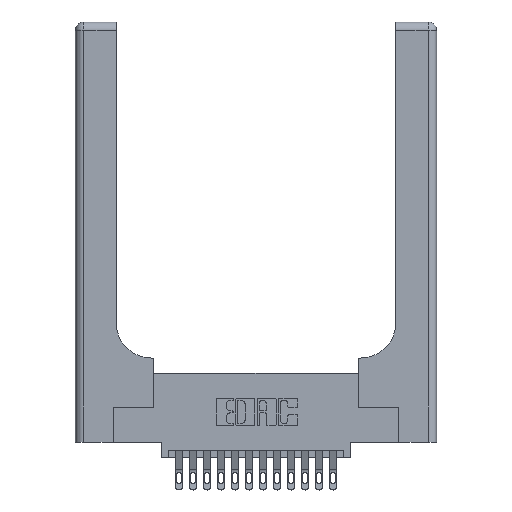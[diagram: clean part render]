
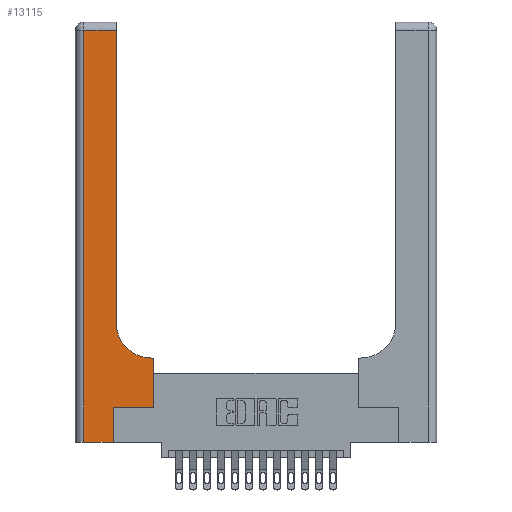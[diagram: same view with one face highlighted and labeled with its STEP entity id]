
A CAD part, top view. The second image highlights one B-rep face of the part: STEP entity #13115.
In plain terms, the highlighted planar face has unit normal (0, 0, 1).
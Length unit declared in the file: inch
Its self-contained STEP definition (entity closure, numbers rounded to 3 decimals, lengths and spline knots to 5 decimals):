
#173 = EDGE_CURVE ( 'NONE', #11766, #14935, #10008, .T. ) ;
#543 = ORIENTED_EDGE ( 'NONE', *, *, #10505, .T. ) ;
#1247 = CARTESIAN_POINT ( 'NONE',  ( 0.5415, 0.85, 0.37 ) ) ;
#1340 = VECTOR ( 'NONE', #4042, 39.37008 ) ;
#1445 = VECTOR ( 'NONE', #12052, 39.37008 ) ;
#2029 = FACE_OUTER_BOUND ( 'NONE', #12552, .T. ) ;
#2255 = EDGE_CURVE ( 'NONE', #11863, #18431, #16213, .T. ) ;
#2437 = CARTESIAN_POINT ( 'NONE',  ( 0.5415, 0.6, 0.37 ) ) ;
#2959 = AXIS2_PLACEMENT_3D ( 'NONE', #1247, #5546, #6904 ) ;
#3194 = CARTESIAN_POINT ( 'NONE',  ( 0., 0., 0.37 ) ) ;
#3254 = EDGE_CURVE ( 'NONE', #19071, #11415, #4834, .T. ) ;
#3651 = EDGE_CURVE ( 'NONE', #17172, #5859, #17070, .T. ) ;
#3893 = DIRECTION ( 'NONE',  ( 0., -1., 0. ) ) ;
#4042 = DIRECTION ( 'NONE',  ( 0., 1., 0. ) ) ;
#4176 = CARTESIAN_POINT ( 'NONE',  ( 0.06, 2.94, 0.37 ) ) ;
#4649 = DIRECTION ( 'NONE',  ( 1., 0., 0. ) ) ;
#4834 = LINE ( 'NONE', #18216, #10853 ) ;
#5546 = DIRECTION ( 'NONE',  ( 0., 0., -1. ) ) ;
#5724 = LINE ( 'NONE', #3194, #14033 ) ;
#5859 = VERTEX_POINT ( 'NONE', #2437 ) ;
#6064 = PLANE ( 'NONE',  #14473 ) ;
#6672 = CARTESIAN_POINT ( 'NONE',  ( 0.269, 0., 0.37 ) ) ;
#6705 = CARTESIAN_POINT ( 'NONE',  ( 0.269, 0.25, 0.37 ) ) ;
#6874 = CARTESIAN_POINT ( 'NONE',  ( 0.06, 3., 0.37 ) ) ;
#6904 = DIRECTION ( 'NONE',  ( 1., 0., 0. ) ) ;
#7171 = DIRECTION ( 'NONE',  ( -1., 0., 0. ) ) ;
#7426 = LINE ( 'NONE', #9111, #1445 ) ;
#9111 = CARTESIAN_POINT ( 'NONE',  ( 0., 2.94, 0.37 ) ) ;
#9123 = LINE ( 'NONE', #15254, #11876 ) ;
#9161 = VERTEX_POINT ( 'NONE', #6672 ) ;
#9186 = CARTESIAN_POINT ( 'NONE',  ( 0.2915, 2.94, 0.37 ) ) ;
#9344 = ORIENTED_EDGE ( 'NONE', *, *, #15703, .T. ) ;
#10008 = LINE ( 'NONE', #6705, #10236 ) ;
#10175 = VECTOR ( 'NONE', #7171, 39.37008 ) ;
#10236 = VECTOR ( 'NONE', #12768, 39.37008 ) ;
#10370 = CIRCLE ( 'NONE', #2959, 0.25 ) ;
#10505 = EDGE_CURVE ( 'NONE', #18431, #9161, #5724, .T. ) ;
#10602 = DIRECTION ( 'NONE',  ( 0., 0., -1. ) ) ;
#10853 = VECTOR ( 'NONE', #18096, 39.37008 ) ;
#11400 = CARTESIAN_POINT ( 'NONE',  ( 0.269, 0.25, 0.37 ) ) ;
#11415 = VERTEX_POINT ( 'NONE', #9186 ) ;
#11676 = ORIENTED_EDGE ( 'NONE', *, *, #13260, .T. ) ;
#11766 = VERTEX_POINT ( 'NONE', #11400 ) ;
#11863 = VERTEX_POINT ( 'NONE', #4176 ) ;
#11876 = VECTOR ( 'NONE', #16754, 39.37008 ) ;
#12052 = DIRECTION ( 'NONE',  ( -1., 0., 0. ) ) ;
#12241 = VECTOR ( 'NONE', #3893, 39.37008 ) ;
#12386 = LINE ( 'NONE', #15886, #1340 ) ;
#12394 = EDGE_CURVE ( 'NONE', #5859, #19071, #10370, .T. ) ;
#12416 = CARTESIAN_POINT ( 'NONE',  ( 0.2915, 0.85, 0.37 ) ) ;
#12552 = EDGE_LOOP ( 'NONE', ( #16445, #13290, #14454, #543, #9344, #18890, #11676, #16638, #16755 ) ) ;
#12768 = DIRECTION ( 'NONE',  ( 1., 0., 0. ) ) ;
#13115 = ADVANCED_FACE ( 'NONE', ( #2029 ), #6064, .F. ) ;
#13260 = EDGE_CURVE ( 'NONE', #14935, #17172, #12386, .T. ) ;
#13290 = ORIENTED_EDGE ( 'NONE', *, *, #17260, .T. ) ;
#13582 = DIRECTION ( 'NONE',  ( -1., 0., 0. ) ) ;
#14033 = VECTOR ( 'NONE', #4649, 39.37008 ) ;
#14454 = ORIENTED_EDGE ( 'NONE', *, *, #2255, .T. ) ;
#14473 = AXIS2_PLACEMENT_3D ( 'NONE', #17962, #10602, #13582 ) ;
#14935 = VERTEX_POINT ( 'NONE', #16597 ) ;
#15254 = CARTESIAN_POINT ( 'NONE',  ( 0.269, 0., 0.37 ) ) ;
#15486 = CARTESIAN_POINT ( 'NONE',  ( 0.06, 0., 0.37 ) ) ;
#15703 = EDGE_CURVE ( 'NONE', #9161, #11766, #9123, .T. ) ;
#15886 = CARTESIAN_POINT ( 'NONE',  ( 0.5585, 0.25, 0.37 ) ) ;
#16213 = LINE ( 'NONE', #6874, #12241 ) ;
#16445 = ORIENTED_EDGE ( 'NONE', *, *, #3254, .T. ) ;
#16597 = CARTESIAN_POINT ( 'NONE',  ( 0.5585, 0.25, 0.37 ) ) ;
#16638 = ORIENTED_EDGE ( 'NONE', *, *, #3651, .T. ) ;
#16754 = DIRECTION ( 'NONE',  ( 0., 1., 0. ) ) ;
#16755 = ORIENTED_EDGE ( 'NONE', *, *, #12394, .T. ) ;
#17070 = LINE ( 'NONE', #18995, #10175 ) ;
#17172 = VERTEX_POINT ( 'NONE', #17807 ) ;
#17260 = EDGE_CURVE ( 'NONE', #11415, #11863, #7426, .T. ) ;
#17807 = CARTESIAN_POINT ( 'NONE',  ( 0.5585, 0.6, 0.37 ) ) ;
#17962 = CARTESIAN_POINT ( 'NONE',  ( 0., 3., 0.37 ) ) ;
#18096 = DIRECTION ( 'NONE',  ( 0., 1., 0. ) ) ;
#18216 = CARTESIAN_POINT ( 'NONE',  ( 0.2915, 3., 0.37 ) ) ;
#18431 = VERTEX_POINT ( 'NONE', #15486 ) ;
#18890 = ORIENTED_EDGE ( 'NONE', *, *, #173, .T. ) ;
#18995 = CARTESIAN_POINT ( 'NONE',  ( 0.2915, 0.6, 0.37 ) ) ;
#19071 = VERTEX_POINT ( 'NONE', #12416 ) ;
